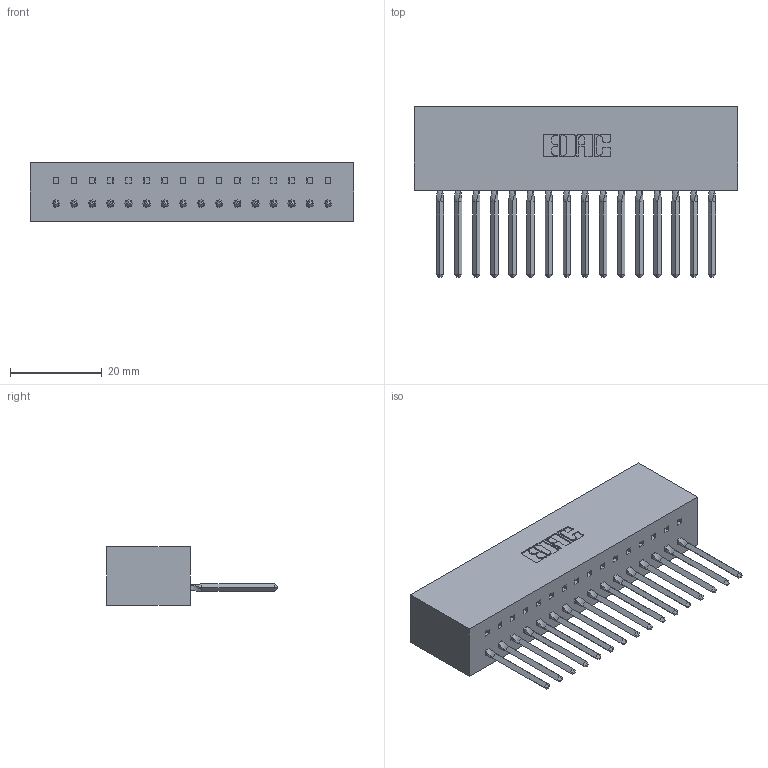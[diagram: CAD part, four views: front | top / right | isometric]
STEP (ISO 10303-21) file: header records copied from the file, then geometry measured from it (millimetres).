
FILE_DESCRIPTION (( 'STEP AP203' ), '1' );
FILE_NAME ('317-016-541-601.STEP', '2020-02-27T15:13:12', ( '' ), ( '' ), 'SwSTEP 2.0', 'SolidWorks 2016', '' );
FILE_SCHEMA (( 'CONFIG_CONTROL_DESIGN' ));
Length unit declared in the file: inch
Products named in the file (3): 317-290-002_541; 317-016-541-601; 317 Part_Lugless
Assembly tree (17 placements, depth 2):
  317-016-541-601
    317 Part_Lugless
    317-290-002_541  x16
Bounding box: 70.61 x 37.34 x 12.7 mm (x, y, z)
Volume: 12357.2 mm3; surface area: 16788.5 mm2
Topology: 17 solids, 17 shells, 2522 faces, 7183 edges, 4670 vertices
Faces by surface type: plane 2034, cylinder 424, bspline 64
Entity records: 27382 total; most frequent: CARTESIAN_POINT 5497, ORIENTED_EDGE 4766, DIRECTION 3887, EDGE_CURVE 2383, LINE 2027, VECTOR 2027, VERTEX_POINT 1580, AXIS2_PLACEMENT_3D 930
